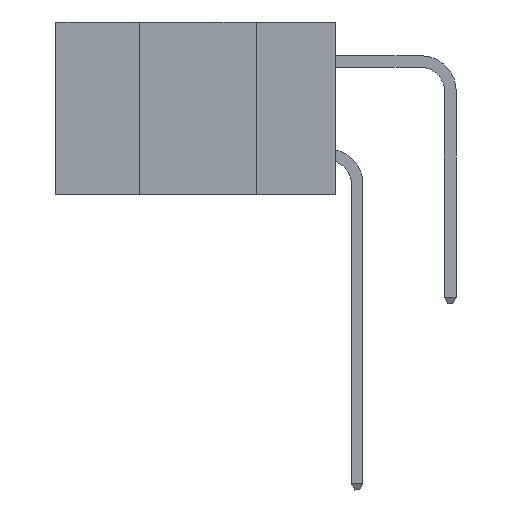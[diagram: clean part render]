
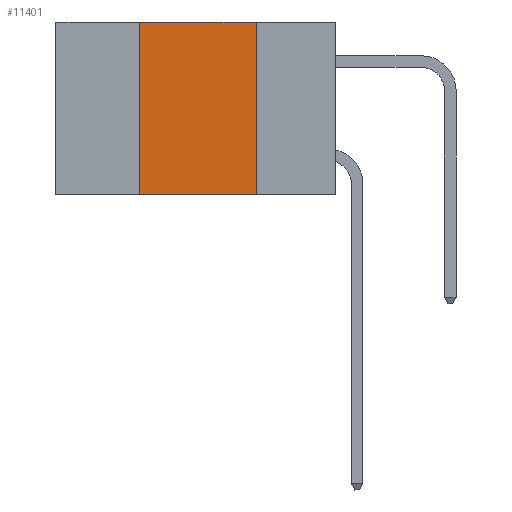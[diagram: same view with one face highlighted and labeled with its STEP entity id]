
A CAD part, left-side view. The second image highlights one B-rep face of the part: STEP entity #11401.
In plain terms, the highlighted planar face has unit normal (-1, 0, 0).
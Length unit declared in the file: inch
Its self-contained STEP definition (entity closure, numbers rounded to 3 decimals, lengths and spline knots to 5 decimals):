
#147 = ORIENTED_EDGE ( 'NONE', *, *, #1081, .F. ) ;
#222 = EDGE_LOOP ( 'NONE', ( #147, #5596, #21791, #17870 ) ) ;
#1081 = EDGE_CURVE ( 'NONE', #20795, #12891, #19274, .T. ) ;
#1427 = VERTEX_POINT ( 'NONE', #3683 ) ;
#1723 = EDGE_CURVE ( 'NONE', #1427, #19024, #14380, .T. ) ;
#2718 = FACE_OUTER_BOUND ( 'NONE', #222, .T. ) ;
#3497 = PLANE ( 'NONE',  #20686 ) ;
#3683 = CARTESIAN_POINT ( 'NONE',  ( 0., 0.42, -0.37 ) ) ;
#5082 = DIRECTION ( 'NONE',  ( 0., -1., 0. ) ) ;
#5562 = DIRECTION ( 'NONE',  ( 0., 0., -1. ) ) ;
#5596 = ORIENTED_EDGE ( 'NONE', *, *, #17835, .F. ) ;
#6279 = CARTESIAN_POINT ( 'NONE',  ( 0., 0.17, -0.37 ) ) ;
#9155 = VECTOR ( 'NONE', #14522, 39.37008 ) ;
#9466 = CARTESIAN_POINT ( 'NONE',  ( 0., 0.6, 0. ) ) ;
#10102 = VECTOR ( 'NONE', #22232, 39.37008 ) ;
#10458 = CARTESIAN_POINT ( 'NONE',  ( 0., 0.6, -0.37 ) ) ;
#10546 = CARTESIAN_POINT ( 'NONE',  ( 0., 0.17, 0. ) ) ;
#10608 = CARTESIAN_POINT ( 'NONE',  ( 0., 0.17, 0. ) ) ;
#11401 = ADVANCED_FACE ( 'NONE', ( #2718 ), #3497, .F. ) ;
#12891 = VERTEX_POINT ( 'NONE', #6279 ) ;
#14380 = LINE ( 'NONE', #22204, #9155 ) ;
#14522 = DIRECTION ( 'NONE',  ( 0., 0., 1. ) ) ;
#15967 = LINE ( 'NONE', #10458, #21093 ) ;
#16122 = VECTOR ( 'NONE', #5082, 39.37008 ) ;
#16728 = LINE ( 'NONE', #20790, #16122 ) ;
#17328 = DIRECTION ( 'NONE',  ( 1., 0., 0. ) ) ;
#17835 = EDGE_CURVE ( 'NONE', #19024, #20795, #16728, .T. ) ;
#17870 = ORIENTED_EDGE ( 'NONE', *, *, #20737, .T. ) ;
#19024 = VERTEX_POINT ( 'NONE', #24381 ) ;
#19274 = LINE ( 'NONE', #10608, #10102 ) ;
#20686 = AXIS2_PLACEMENT_3D ( 'NONE', #9466, #17328, #5562 ) ;
#20737 = EDGE_CURVE ( 'NONE', #1427, #12891, #15967, .T. ) ;
#20790 = CARTESIAN_POINT ( 'NONE',  ( 0., 0.6, 0. ) ) ;
#20795 = VERTEX_POINT ( 'NONE', #10546 ) ;
#21093 = VECTOR ( 'NONE', #22090, 39.37008 ) ;
#21791 = ORIENTED_EDGE ( 'NONE', *, *, #1723, .F. ) ;
#22090 = DIRECTION ( 'NONE',  ( 0., -1., 0. ) ) ;
#22204 = CARTESIAN_POINT ( 'NONE',  ( 0., 0.42, 0. ) ) ;
#22232 = DIRECTION ( 'NONE',  ( 0., 0., -1. ) ) ;
#24381 = CARTESIAN_POINT ( 'NONE',  ( 0., 0.42, 0. ) ) ;
